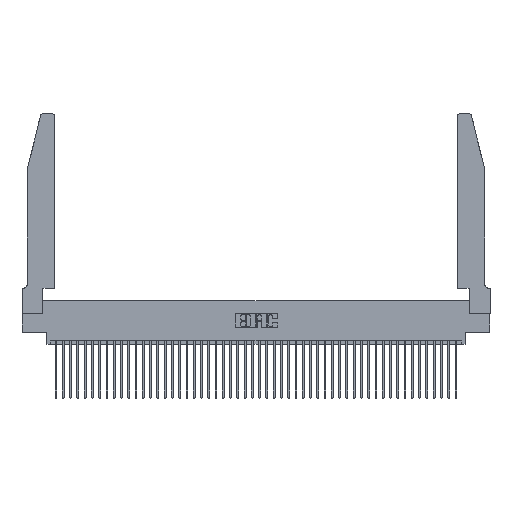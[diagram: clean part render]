
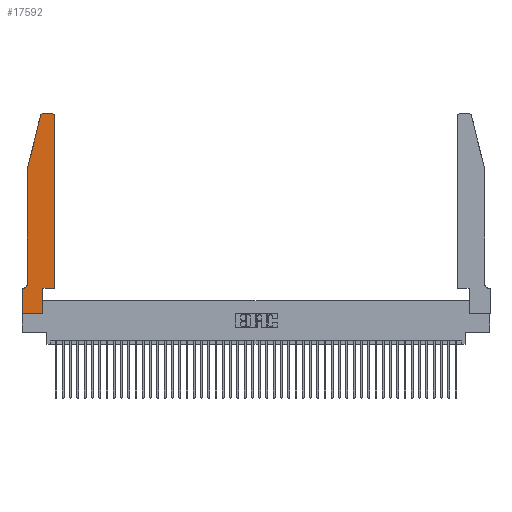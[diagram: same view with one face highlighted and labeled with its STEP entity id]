
A CAD part, top view. The second image highlights one B-rep face of the part: STEP entity #17592.
In plain terms, the highlighted planar face has unit normal (0, 0, 1).
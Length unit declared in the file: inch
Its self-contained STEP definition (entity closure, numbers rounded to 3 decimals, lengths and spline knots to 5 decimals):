
#188 = VECTOR ( 'NONE', #13088, 39.37008 ) ;
#1611 = EDGE_CURVE ( 'NONE', #3707, #11614, #42749, .T. ) ;
#2258 = VECTOR ( 'NONE', #2487, 39.37008 ) ;
#2387 = CARTESIAN_POINT ( 'NONE',  ( 0.4505, 2.72, 0.37 ) ) ;
#2487 = DIRECTION ( 'NONE',  ( 1., 0., 0. ) ) ;
#2661 = VERTEX_POINT ( 'NONE', #33531 ) ;
#3707 = VERTEX_POINT ( 'NONE', #16091 ) ;
#3767 = EDGE_CURVE ( 'NONE', #19384, #42396, #25511, .T. ) ;
#4204 = CARTESIAN_POINT ( 'NONE',  ( 0., 0., 0.37 ) ) ;
#4612 = VECTOR ( 'NONE', #34581, 39.37008 ) ;
#5701 = CIRCLE ( 'NONE', #26824, 0.07 ) ;
#6287 = VECTOR ( 'NONE', #27068, 39.37008 ) ;
#7022 = VECTOR ( 'NONE', #20563, 39.37008 ) ;
#7139 = DIRECTION ( 'NONE',  ( 0., 0., 1. ) ) ;
#7540 = AXIS2_PLACEMENT_3D ( 'NONE', #39732, #7139, #22324 ) ;
#7622 = EDGE_CURVE ( 'NONE', #9942, #12116, #17503, .T. ) ;
#8269 = CARTESIAN_POINT ( 'NONE',  ( 0.284, 2.72, 0.37 ) ) ;
#8305 = DIRECTION ( 'NONE',  ( 1., 0., 0. ) ) ;
#8485 = DIRECTION ( 'NONE',  ( 1., 0., 0. ) ) ;
#9235 = CARTESIAN_POINT ( 'NONE',  ( 0., 0., 0.37 ) ) ;
#9789 = CARTESIAN_POINT ( 'NONE',  ( 0.0755, 0.35, 0.37 ) ) ;
#9942 = VERTEX_POINT ( 'NONE', #34292 ) ;
#10253 = VECTOR ( 'NONE', #38907, 39.37008 ) ;
#10524 = DIRECTION ( 'NONE',  ( 0., 0., -1. ) ) ;
#11479 = ORIENTED_EDGE ( 'NONE', *, *, #35616, .T. ) ;
#11480 = DIRECTION ( 'NONE',  ( 0., -1., 0. ) ) ;
#11533 = VECTOR ( 'NONE', #11480, 39.37008 ) ;
#11614 = VERTEX_POINT ( 'NONE', #40632 ) ;
#11978 = EDGE_CURVE ( 'NONE', #42396, #3707, #36266, .T. ) ;
#12116 = VERTEX_POINT ( 'NONE', #42797 ) ;
#12162 = VERTEX_POINT ( 'NONE', #34944 ) ;
#13088 = DIRECTION ( 'NONE',  ( -1., 0., 0. ) ) ;
#14177 = DIRECTION ( 'NONE',  ( -1., 0., 0. ) ) ;
#14264 = LINE ( 'NONE', #16392, #4612 ) ;
#14667 = ORIENTED_EDGE ( 'NONE', *, *, #3767, .T. ) ;
#14948 = DIRECTION ( 'NONE',  ( 0., 0., 1. ) ) ;
#15351 = CARTESIAN_POINT ( 'NONE',  ( 0.2605, 2.75, 0.37 ) ) ;
#16091 = CARTESIAN_POINT ( 'NONE',  ( 0.0755, 2., 0.37 ) ) ;
#16359 = VECTOR ( 'NONE', #8305, 39.37008 ) ;
#16392 = CARTESIAN_POINT ( 'NONE',  ( 0.4505, 0.35, 0.37 ) ) ;
#17105 = CARTESIAN_POINT ( 'NONE',  ( 0.284, 2.75, 0.37 ) ) ;
#17503 = LINE ( 'NONE', #30307, #16359 ) ;
#17592 = ADVANCED_FACE ( 'NONE', ( #42010 ), #39585, .T. ) ;
#18097 = EDGE_LOOP ( 'NONE', ( #26357, #14667, #30520, #40414, #36720, #18759, #29406, #38830, #11479, #32602, #39881, #33743 ) ) ;
#18759 = ORIENTED_EDGE ( 'NONE', *, *, #32652, .T. ) ;
#18768 = VECTOR ( 'NONE', #43573, 39.37008 ) ;
#19384 = VERTEX_POINT ( 'NONE', #17105 ) ;
#19793 = VERTEX_POINT ( 'NONE', #2387 ) ;
#20563 = DIRECTION ( 'NONE',  ( 0., -1., 0. ) ) ;
#22218 = CARTESIAN_POINT ( 'NONE',  ( 0.4205, 2.75, 0.37 ) ) ;
#22324 = DIRECTION ( 'NONE',  ( 1., 0., 0. ) ) ;
#24420 = LINE ( 'NONE', #45467, #6287 ) ;
#25002 = AXIS2_PLACEMENT_3D ( 'NONE', #37062, #14948, #8485 ) ;
#25243 = EDGE_CURVE ( 'NONE', #32937, #19384, #25623, .T. ) ;
#25511 = CIRCLE ( 'NONE', #39909, 0.03 ) ;
#25623 = LINE ( 'NONE', #15351, #18768 ) ;
#26357 = ORIENTED_EDGE ( 'NONE', *, *, #25243, .T. ) ;
#26417 = EDGE_CURVE ( 'NONE', #19793, #32937, #40553, .T. ) ;
#26824 = AXIS2_PLACEMENT_3D ( 'NONE', #32236, #10524, #14177 ) ;
#27068 = DIRECTION ( 'NONE',  ( 0., 1., 0. ) ) ;
#27302 = DIRECTION ( 'NONE',  ( 0., 0., 1. ) ) ;
#27670 = EDGE_CURVE ( 'NONE', #2661, #29943, #37002, .T. ) ;
#28264 = VERTEX_POINT ( 'NONE', #43383 ) ;
#28890 = LINE ( 'NONE', #31170, #2258 ) ;
#29164 = EDGE_CURVE ( 'NONE', #12116, #19793, #14264, .T. ) ;
#29406 = ORIENTED_EDGE ( 'NONE', *, *, #27670, .T. ) ;
#29943 = VERTEX_POINT ( 'NONE', #9235 ) ;
#30307 = CARTESIAN_POINT ( 'NONE',  ( 0.4505, 0.35, 0.37 ) ) ;
#30520 = ORIENTED_EDGE ( 'NONE', *, *, #11978, .T. ) ;
#31170 = CARTESIAN_POINT ( 'NONE',  ( 0., 0., 0.37 ) ) ;
#32236 = CARTESIAN_POINT ( 'NONE',  ( 0.0055, 0.42, 0.37 ) ) ;
#32602 = ORIENTED_EDGE ( 'NONE', *, *, #7622, .T. ) ;
#32652 = EDGE_CURVE ( 'NONE', #28264, #2661, #37022, .T. ) ;
#32937 = VERTEX_POINT ( 'NONE', #22218 ) ;
#33531 = CARTESIAN_POINT ( 'NONE',  ( 0., 0.35, 0.37 ) ) ;
#33743 = ORIENTED_EDGE ( 'NONE', *, *, #26417, .T. ) ;
#34292 = CARTESIAN_POINT ( 'NONE',  ( 0.2865, 0.35, 0.37 ) ) ;
#34581 = DIRECTION ( 'NONE',  ( 0., 1., 0. ) ) ;
#34944 = CARTESIAN_POINT ( 'NONE',  ( 0.2865, 0., 0.37 ) ) ;
#35616 = EDGE_CURVE ( 'NONE', #12162, #9942, #24420, .T. ) ;
#35829 = EDGE_CURVE ( 'NONE', #29943, #12162, #28890, .T. ) ;
#35850 = CARTESIAN_POINT ( 'NONE',  ( 0.25487, 2.72718, 0.37 ) ) ;
#35987 = EDGE_CURVE ( 'NONE', #11614, #28264, #5701, .T. ) ;
#36266 = LINE ( 'NONE', #38281, #10253 ) ;
#36720 = ORIENTED_EDGE ( 'NONE', *, *, #35987, .T. ) ;
#37002 = LINE ( 'NONE', #4204, #11533 ) ;
#37022 = LINE ( 'NONE', #9789, #188 ) ;
#37062 = CARTESIAN_POINT ( 'NONE',  ( 0.4205, 2.72, 0.37 ) ) ;
#38281 = CARTESIAN_POINT ( 'NONE',  ( 0.0755, 2., 0.37 ) ) ;
#38830 = ORIENTED_EDGE ( 'NONE', *, *, #35829, .T. ) ;
#38907 = DIRECTION ( 'NONE',  ( -0.239, -0.971, 0. ) ) ;
#39585 = PLANE ( 'NONE',  #7540 ) ;
#39732 = CARTESIAN_POINT ( 'NONE',  ( 0., 0.35, 0.37 ) ) ;
#39752 = DIRECTION ( 'NONE',  ( 1., 0., 0. ) ) ;
#39881 = ORIENTED_EDGE ( 'NONE', *, *, #29164, .T. ) ;
#39909 = AXIS2_PLACEMENT_3D ( 'NONE', #8269, #27302, #39752 ) ;
#40414 = ORIENTED_EDGE ( 'NONE', *, *, #1611, .T. ) ;
#40553 = CIRCLE ( 'NONE', #25002, 0.03 ) ;
#40632 = CARTESIAN_POINT ( 'NONE',  ( 0.0755, 0.42, 0.37 ) ) ;
#42010 = FACE_OUTER_BOUND ( 'NONE', #18097, .T. ) ;
#42396 = VERTEX_POINT ( 'NONE', #35850 ) ;
#42575 = CARTESIAN_POINT ( 'NONE',  ( 0.0755, 2., 0.37 ) ) ;
#42749 = LINE ( 'NONE', #42575, #7022 ) ;
#42797 = CARTESIAN_POINT ( 'NONE',  ( 0.4505, 0.35, 0.37 ) ) ;
#43383 = CARTESIAN_POINT ( 'NONE',  ( 0.0055, 0.35, 0.37 ) ) ;
#43573 = DIRECTION ( 'NONE',  ( -1., 0., 0. ) ) ;
#45467 = CARTESIAN_POINT ( 'NONE',  ( 0.2865, 0.35, 0.37 ) ) ;
